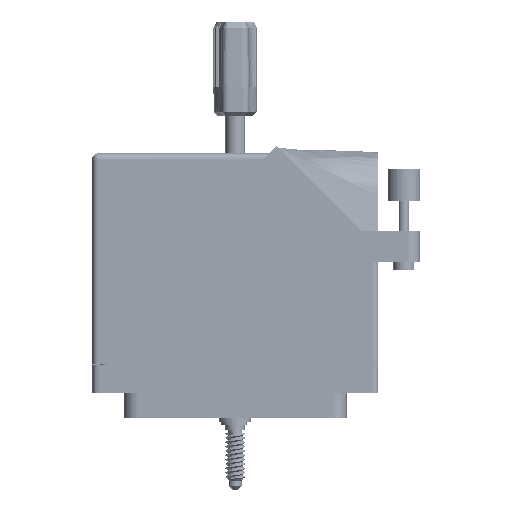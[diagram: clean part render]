
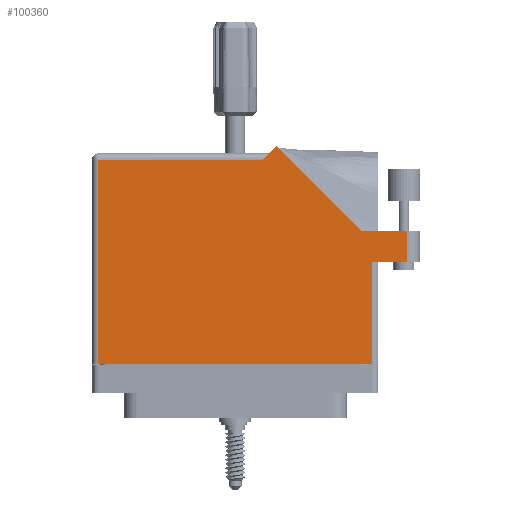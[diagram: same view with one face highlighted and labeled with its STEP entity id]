
A CAD part, front view. The second image highlights one B-rep face of the part: STEP entity #100360.
In plain terms, the highlighted face is planar.
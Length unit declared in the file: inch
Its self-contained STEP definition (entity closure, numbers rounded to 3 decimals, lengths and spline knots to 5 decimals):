
#878 = VECTOR ( 'NONE', #56740, 39.37008 ) ;
#1336 = LINE ( 'NONE', #59233, #62635 ) ;
#2859 = CARTESIAN_POINT ( 'NONE',  ( 1.3775, 0.88, 0.765 ) ) ;
#3179 = AXIS2_PLACEMENT_3D ( 'NONE', #83766, #18459, #75470 ) ;
#3768 = DIRECTION ( 'NONE',  ( 1., 0., 0. ) ) ;
#3801 = VERTEX_POINT ( 'NONE', #39436 ) ;
#4901 = CARTESIAN_POINT ( 'NONE',  ( 1.3155, 0.88, 0.765 ) ) ;
#5068 = VERTEX_POINT ( 'NONE', #77214 ) ;
#5284 = EDGE_CURVE ( 'NONE', #89979, #17593, #8037, .T. ) ;
#5491 = VECTOR ( 'NONE', #50928, 39.37008 ) ;
#5740 = EDGE_LOOP ( 'NONE', ( #5910, #86309, #20143, #63520, #29756, #6349, #87443, #48486, #83027 ) ) ;
#5910 = ORIENTED_EDGE ( 'NONE', *, *, #7690, .T. ) ;
#6349 = ORIENTED_EDGE ( 'NONE', *, *, #87145, .T. ) ;
#7690 = EDGE_CURVE ( 'NONE', #35738, #3801, #75206, .T. ) ;
#8037 = LINE ( 'NONE', #34551, #5491 ) ;
#8176 = CARTESIAN_POINT ( 'NONE',  ( -1.3155, 1.868, 0.765 ) ) ;
#8425 = VECTOR ( 'NONE', #72306, 39.37008 ) ;
#8933 = VECTOR ( 'NONE', #99051, 39.37008 ) ;
#11317 = PLANE ( 'NONE',  #3179 ) ;
#17052 = LINE ( 'NONE', #4901, #51522 ) ;
#17593 = VERTEX_POINT ( 'NONE', #37094 ) ;
#18459 = DIRECTION ( 'NONE',  ( 0., 0., -1. ) ) ;
#19249 = DIRECTION ( 'NONE',  ( 1., 0., 0. ) ) ;
#20143 = ORIENTED_EDGE ( 'NONE', *, *, #28307, .T. ) ;
#21321 = DIRECTION ( 'NONE',  ( 0., 1., 0. ) ) ;
#28307 = EDGE_CURVE ( 'NONE', #5068, #98597, #1336, .T. ) ;
#29756 = ORIENTED_EDGE ( 'NONE', *, *, #5284, .T. ) ;
#34551 = CARTESIAN_POINT ( 'NONE',  ( 0.3275, 1.93, 0.765 ) ) ;
#35628 = VECTOR ( 'NONE', #89862, 39.37008 ) ;
#35738 = VERTEX_POINT ( 'NONE', #102625 ) ;
#37094 = CARTESIAN_POINT ( 'NONE',  ( 0.2655, 1.868, 0.765 ) ) ;
#39436 = CARTESIAN_POINT ( 'NONE',  ( 1.6525, 0.88, 0.765 ) ) ;
#41792 = CARTESIAN_POINT ( 'NONE',  ( 1.21192, 1.187, 0.765 ) ) ;
#48486 = ORIENTED_EDGE ( 'NONE', *, *, #64666, .T. ) ;
#48556 = CARTESIAN_POINT ( 'NONE',  ( -1.3775, 1.868, 0.765 ) ) ;
#50928 = DIRECTION ( 'NONE',  ( -0.707, -0.707, 0. ) ) ;
#51522 = VECTOR ( 'NONE', #21321, 39.37008 ) ;
#54077 = VERTEX_POINT ( 'NONE', #8176 ) ;
#54812 = VECTOR ( 'NONE', #19249, 39.37008 ) ;
#54905 = CARTESIAN_POINT ( 'NONE',  ( 0.39821, 2.00071, 0.765 ) ) ;
#56740 = DIRECTION ( 'NONE',  ( -1., 0., 0. ) ) ;
#59233 = CARTESIAN_POINT ( 'NONE',  ( 1.7775, 1.187, 0.765 ) ) ;
#62635 = VECTOR ( 'NONE', #69920, 39.37008 ) ;
#62714 = CARTESIAN_POINT ( 'NONE',  ( 1.6525, 1.187, 0.765 ) ) ;
#62988 = FACE_OUTER_BOUND ( 'NONE', #5740, .T. ) ;
#63520 = ORIENTED_EDGE ( 'NONE', *, *, #96550, .T. ) ;
#64666 = EDGE_CURVE ( 'NONE', #83971, #69541, #71202, .T. ) ;
#68766 = LINE ( 'NONE', #81240, #35628 ) ;
#69541 = VERTEX_POINT ( 'NONE', #96318 ) ;
#69718 = CARTESIAN_POINT ( 'NONE',  ( -1.3775, -0.1, 0.765 ) ) ;
#69920 = DIRECTION ( 'NONE',  ( -1., 0., 0. ) ) ;
#71202 = LINE ( 'NONE', #69718, #98181 ) ;
#72306 = DIRECTION ( 'NONE',  ( 0., 1., 0. ) ) ;
#72530 = CARTESIAN_POINT ( 'NONE',  ( -1.3155, -0.1, 0.765 ) ) ;
#73322 = EDGE_CURVE ( 'NONE', #54077, #83971, #68766, .T. ) ;
#75206 = LINE ( 'NONE', #2859, #54812 ) ;
#75470 = DIRECTION ( 'NONE',  ( -1., 0., 0. ) ) ;
#77021 = CARTESIAN_POINT ( 'NONE',  ( 1.21192, 1.187, 0.765 ) ) ;
#77214 = CARTESIAN_POINT ( 'NONE',  ( 1.6525, 1.187, 0.765 ) ) ;
#79986 = LINE ( 'NONE', #48556, #878 ) ;
#81240 = CARTESIAN_POINT ( 'NONE',  ( -1.3155, -0.1, 0.765 ) ) ;
#81726 = LINE ( 'NONE', #41792, #8933 ) ;
#83027 = ORIENTED_EDGE ( 'NONE', *, *, #101192, .T. ) ;
#83766 = CARTESIAN_POINT ( 'NONE',  ( -1.3775, 1.93, 0.765 ) ) ;
#83971 = VERTEX_POINT ( 'NONE', #72530 ) ;
#86309 = ORIENTED_EDGE ( 'NONE', *, *, #90312, .T. ) ;
#87145 = EDGE_CURVE ( 'NONE', #17593, #54077, #79986, .T. ) ;
#87443 = ORIENTED_EDGE ( 'NONE', *, *, #73322, .T. ) ;
#89862 = DIRECTION ( 'NONE',  ( 0., -1., 0. ) ) ;
#89979 = VERTEX_POINT ( 'NONE', #54905 ) ;
#90312 = EDGE_CURVE ( 'NONE', #3801, #5068, #104269, .T. ) ;
#96318 = CARTESIAN_POINT ( 'NONE',  ( 1.3155, -0.1, 0.765 ) ) ;
#96550 = EDGE_CURVE ( 'NONE', #98597, #89979, #81726, .T. ) ;
#98181 = VECTOR ( 'NONE', #3768, 39.37008 ) ;
#98597 = VERTEX_POINT ( 'NONE', #77021 ) ;
#99051 = DIRECTION ( 'NONE',  ( -0.707, 0.707, 0. ) ) ;
#100360 = ADVANCED_FACE ( 'NONE', ( #62988 ), #11317, .F. ) ;
#101192 = EDGE_CURVE ( 'NONE', #69541, #35738, #17052, .T. ) ;
#102625 = CARTESIAN_POINT ( 'NONE',  ( 1.3155, 0.88, 0.765 ) ) ;
#104269 = LINE ( 'NONE', #62714, #8425 ) ;
